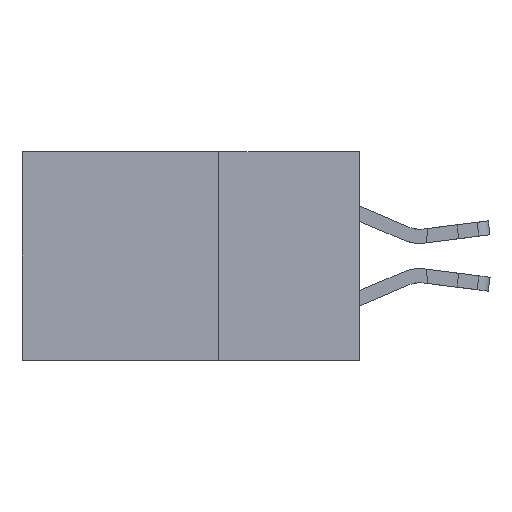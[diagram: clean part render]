
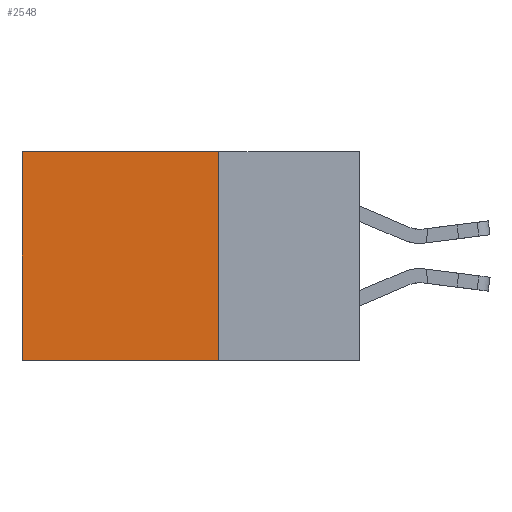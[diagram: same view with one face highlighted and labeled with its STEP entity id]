
A CAD part, left-side view. The second image highlights one B-rep face of the part: STEP entity #2548.
In plain terms, the highlighted planar face has unit normal (-1, 0, 0).
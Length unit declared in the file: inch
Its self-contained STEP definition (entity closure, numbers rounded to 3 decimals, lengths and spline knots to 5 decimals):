
#7 = CARTESIAN_POINT ( 'NONE',  ( 0.2875, 0.25, -0.37 ) ) ;
#661 = CARTESIAN_POINT ( 'NONE',  ( 0.2875, 0.6, -0.37 ) ) ;
#1223 = CARTESIAN_POINT ( 'NONE',  ( 0.2875, 0.25, 0. ) ) ;
#1262 = CARTESIAN_POINT ( 'NONE',  ( 0.2875, 0.6, 0. ) ) ;
#1556 = VERTEX_POINT ( 'NONE', #661 ) ;
#2247 = EDGE_CURVE ( 'NONE', #24764, #1556, #24876, .T. ) ;
#2548 = ADVANCED_FACE ( 'NONE', ( #18958 ), #22549, .F. ) ;
#3142 = VERTEX_POINT ( 'NONE', #9208 ) ;
#4713 = ORIENTED_EDGE ( 'NONE', *, *, #18167, .T. ) ;
#5695 = LINE ( 'NONE', #1262, #7042 ) ;
#7042 = VECTOR ( 'NONE', #16131, 39.37008 ) ;
#8773 = CARTESIAN_POINT ( 'NONE',  ( 0.2875, 0.25, -0.37 ) ) ;
#9208 = CARTESIAN_POINT ( 'NONE',  ( 0.2875, 0.6, 0. ) ) ;
#9361 = VERTEX_POINT ( 'NONE', #18359 ) ;
#9408 = VECTOR ( 'NONE', #9499, 39.37008 ) ;
#9499 = DIRECTION ( 'NONE',  ( 0., 0., -1. ) ) ;
#9883 = DIRECTION ( 'NONE',  ( 0., 0., -1. ) ) ;
#10040 = VECTOR ( 'NONE', #16194, 39.37008 ) ;
#12895 = EDGE_CURVE ( 'NONE', #9361, #24764, #26901, .T. ) ;
#13781 = AXIS2_PLACEMENT_3D ( 'NONE', #22274, #24447, #9883 ) ;
#14148 = ORIENTED_EDGE ( 'NONE', *, *, #27342, .T. ) ;
#15679 = LINE ( 'NONE', #1223, #10040 ) ;
#16131 = DIRECTION ( 'NONE',  ( 0., 0., -1. ) ) ;
#16194 = DIRECTION ( 'NONE',  ( 0., 1., 0. ) ) ;
#18167 = EDGE_CURVE ( 'NONE', #3142, #1556, #5695, .T. ) ;
#18359 = CARTESIAN_POINT ( 'NONE',  ( 0.2875, 0.25, 0. ) ) ;
#18958 = FACE_OUTER_BOUND ( 'NONE', #24061, .T. ) ;
#19150 = ORIENTED_EDGE ( 'NONE', *, *, #12895, .F. ) ;
#21003 = ORIENTED_EDGE ( 'NONE', *, *, #2247, .F. ) ;
#21611 = DIRECTION ( 'NONE',  ( 0., 1., 0. ) ) ;
#22068 = CARTESIAN_POINT ( 'NONE',  ( 0.2875, 0.25, 0. ) ) ;
#22274 = CARTESIAN_POINT ( 'NONE',  ( 0.2875, 0.25, 0. ) ) ;
#22549 = PLANE ( 'NONE',  #13781 ) ;
#24061 = EDGE_LOOP ( 'NONE', ( #4713, #21003, #19150, #14148 ) ) ;
#24177 = VECTOR ( 'NONE', #21611, 39.37008 ) ;
#24447 = DIRECTION ( 'NONE',  ( 1., 0., 0. ) ) ;
#24764 = VERTEX_POINT ( 'NONE', #7 ) ;
#24876 = LINE ( 'NONE', #8773, #24177 ) ;
#26901 = LINE ( 'NONE', #22068, #9408 ) ;
#27342 = EDGE_CURVE ( 'NONE', #9361, #3142, #15679, .T. ) ;
